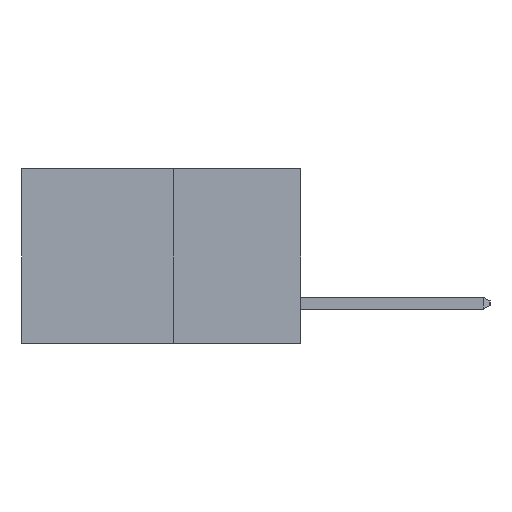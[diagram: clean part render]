
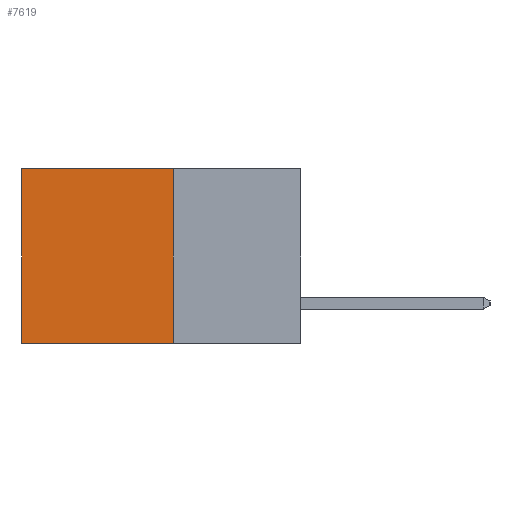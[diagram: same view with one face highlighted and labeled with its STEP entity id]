
A CAD part, left-side view. The second image highlights one B-rep face of the part: STEP entity #7619.
In plain terms, the highlighted planar face has unit normal (-1, 0, 0).
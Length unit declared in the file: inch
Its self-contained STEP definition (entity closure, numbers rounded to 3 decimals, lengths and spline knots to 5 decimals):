
#27 = DIRECTION ( 'NONE',  ( 0., 0., -1. ) ) ;
#254 = EDGE_CURVE ( 'NONE', #1764, #928, #3574, .T. ) ;
#314 = CARTESIAN_POINT ( 'NONE',  ( 0.277, 0.27, 0. ) ) ;
#361 = VECTOR ( 'NONE', #27, 39.37008 ) ;
#737 = FACE_OUTER_BOUND ( 'NONE', #780, .T. ) ;
#780 = EDGE_LOOP ( 'NONE', ( #10010, #12215, #7338, #6567 ) ) ;
#790 = LINE ( 'NONE', #9079, #5577 ) ;
#928 = VERTEX_POINT ( 'NONE', #8203 ) ;
#1195 = CARTESIAN_POINT ( 'NONE',  ( 0.277, 0.27, -0.37 ) ) ;
#1713 = VECTOR ( 'NONE', #10124, 39.37008 ) ;
#1764 = VERTEX_POINT ( 'NONE', #1195 ) ;
#1918 = VERTEX_POINT ( 'NONE', #314 ) ;
#2005 = EDGE_CURVE ( 'NONE', #1918, #1764, #790, .T. ) ;
#3294 = LINE ( 'NONE', #13158, #361 ) ;
#3458 = AXIS2_PLACEMENT_3D ( 'NONE', #10103, #9625, #9623 ) ;
#3574 = LINE ( 'NONE', #13737, #6102 ) ;
#4319 = DIRECTION ( 'NONE',  ( 0., 1., 0. ) ) ;
#5577 = VECTOR ( 'NONE', #12643, 39.37008 ) ;
#5653 = VERTEX_POINT ( 'NONE', #9041 ) ;
#6102 = VECTOR ( 'NONE', #4319, 39.37008 ) ;
#6497 = EDGE_CURVE ( 'NONE', #1918, #5653, #7162, .T. ) ;
#6567 = ORIENTED_EDGE ( 'NONE', *, *, #6497, .T. ) ;
#7162 = LINE ( 'NONE', #10076, #1713 ) ;
#7338 = ORIENTED_EDGE ( 'NONE', *, *, #2005, .F. ) ;
#7619 = ADVANCED_FACE ( 'NONE', ( #737 ), #9929, .F. ) ;
#8203 = CARTESIAN_POINT ( 'NONE',  ( 0.277, 0.59, -0.37 ) ) ;
#8528 = EDGE_CURVE ( 'NONE', #5653, #928, #3294, .T. ) ;
#9041 = CARTESIAN_POINT ( 'NONE',  ( 0.277, 0.59, 0. ) ) ;
#9079 = CARTESIAN_POINT ( 'NONE',  ( 0.277, 0.27, -0.37 ) ) ;
#9623 = DIRECTION ( 'NONE',  ( 0., 0., -1. ) ) ;
#9625 = DIRECTION ( 'NONE',  ( 1., 0., 0. ) ) ;
#9929 = PLANE ( 'NONE',  #3458 ) ;
#10010 = ORIENTED_EDGE ( 'NONE', *, *, #8528, .T. ) ;
#10076 = CARTESIAN_POINT ( 'NONE',  ( 0.277, 0.27, 0. ) ) ;
#10103 = CARTESIAN_POINT ( 'NONE',  ( 0.277, 0.27, -0.37 ) ) ;
#10124 = DIRECTION ( 'NONE',  ( 0., 1., 0. ) ) ;
#12215 = ORIENTED_EDGE ( 'NONE', *, *, #254, .F. ) ;
#12643 = DIRECTION ( 'NONE',  ( 0., 0., -1. ) ) ;
#13158 = CARTESIAN_POINT ( 'NONE',  ( 0.277, 0.59, -0.37 ) ) ;
#13737 = CARTESIAN_POINT ( 'NONE',  ( 0.277, 0.27, -0.37 ) ) ;
